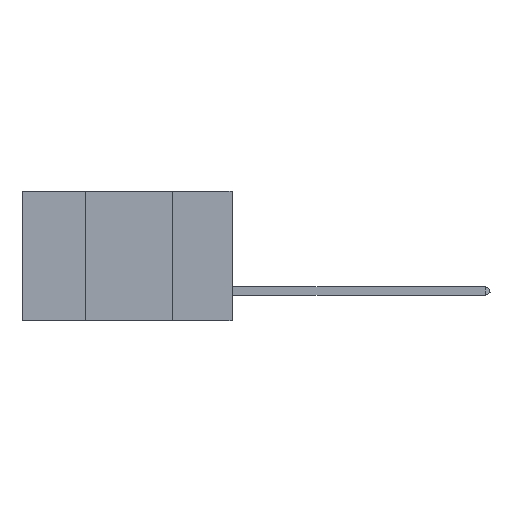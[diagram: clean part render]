
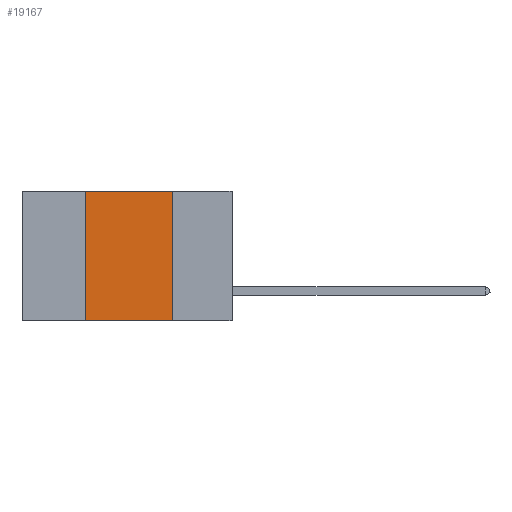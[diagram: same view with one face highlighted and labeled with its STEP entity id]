
A CAD part, left-side view. The second image highlights one B-rep face of the part: STEP entity #19167.
In plain terms, the highlighted planar face has unit normal (-1, 0, 0).
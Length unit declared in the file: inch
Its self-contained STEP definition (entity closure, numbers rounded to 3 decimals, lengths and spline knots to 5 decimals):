
#1028 = PLANE ( 'NONE',  #10625 ) ;
#1162 = DIRECTION ( 'NONE',  ( 1., 0., 0. ) ) ;
#1398 = CARTESIAN_POINT ( 'NONE',  ( 0., 0.17, 0. ) ) ;
#1545 = VERTEX_POINT ( 'NONE', #5917 ) ;
#2694 = VERTEX_POINT ( 'NONE', #8479 ) ;
#3470 = ORIENTED_EDGE ( 'NONE', *, *, #10929, .T. ) ;
#4088 = CARTESIAN_POINT ( 'NONE',  ( 0., 0.6, 0. ) ) ;
#4625 = DIRECTION ( 'NONE',  ( 0., -1., 0. ) ) ;
#4709 = LINE ( 'NONE', #10083, #16916 ) ;
#4797 = EDGE_LOOP ( 'NONE', ( #13629, #10816, #5217, #3470 ) ) ;
#4885 = DIRECTION ( 'NONE',  ( 0., 0., 1. ) ) ;
#5217 = ORIENTED_EDGE ( 'NONE', *, *, #17411, .F. ) ;
#5917 = CARTESIAN_POINT ( 'NONE',  ( 0., 0.17, -0.37 ) ) ;
#7109 = DIRECTION ( 'NONE',  ( 0., -1., 0. ) ) ;
#7470 = VECTOR ( 'NONE', #8876, 39.37008 ) ;
#7859 = VERTEX_POINT ( 'NONE', #1398 ) ;
#8479 = CARTESIAN_POINT ( 'NONE',  ( 0., 0.42, -0.37 ) ) ;
#8699 = LINE ( 'NONE', #19906, #7470 ) ;
#8876 = DIRECTION ( 'NONE',  ( 0., 0., -1. ) ) ;
#9827 = VECTOR ( 'NONE', #4885, 39.37008 ) ;
#10083 = CARTESIAN_POINT ( 'NONE',  ( 0., 0.6, -0.37 ) ) ;
#10625 = AXIS2_PLACEMENT_3D ( 'NONE', #4088, #1162, #18515 ) ;
#10816 = ORIENTED_EDGE ( 'NONE', *, *, #14042, .F. ) ;
#10929 = EDGE_CURVE ( 'NONE', #2694, #1545, #4709, .T. ) ;
#10939 = VECTOR ( 'NONE', #4625, 39.37008 ) ;
#12683 = CARTESIAN_POINT ( 'NONE',  ( 0., 0.6, 0. ) ) ;
#12870 = CARTESIAN_POINT ( 'NONE',  ( 0., 0.42, 0. ) ) ;
#13629 = ORIENTED_EDGE ( 'NONE', *, *, #14514, .F. ) ;
#14012 = FACE_OUTER_BOUND ( 'NONE', #4797, .T. ) ;
#14042 = EDGE_CURVE ( 'NONE', #17120, #7859, #18662, .T. ) ;
#14514 = EDGE_CURVE ( 'NONE', #7859, #1545, #8699, .T. ) ;
#16075 = LINE ( 'NONE', #12870, #9827 ) ;
#16916 = VECTOR ( 'NONE', #7109, 39.37008 ) ;
#17120 = VERTEX_POINT ( 'NONE', #19884 ) ;
#17411 = EDGE_CURVE ( 'NONE', #2694, #17120, #16075, .T. ) ;
#18515 = DIRECTION ( 'NONE',  ( 0., 0., -1. ) ) ;
#18662 = LINE ( 'NONE', #12683, #10939 ) ;
#19167 = ADVANCED_FACE ( 'NONE', ( #14012 ), #1028, .F. ) ;
#19884 = CARTESIAN_POINT ( 'NONE',  ( 0., 0.42, 0. ) ) ;
#19906 = CARTESIAN_POINT ( 'NONE',  ( 0., 0.17, 0. ) ) ;
